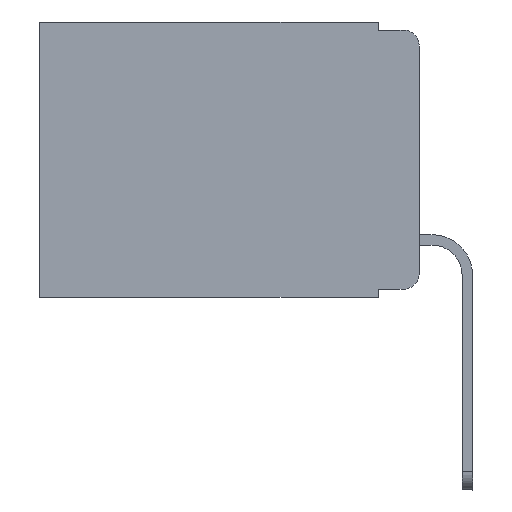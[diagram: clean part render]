
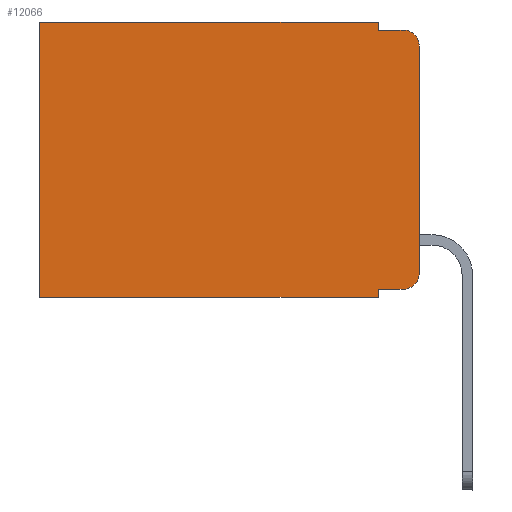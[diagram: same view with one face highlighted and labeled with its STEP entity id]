
A CAD part, left-side view. The second image highlights one B-rep face of the part: STEP entity #12066.
In plain terms, the highlighted planar face has unit normal (-1, 0, 0).
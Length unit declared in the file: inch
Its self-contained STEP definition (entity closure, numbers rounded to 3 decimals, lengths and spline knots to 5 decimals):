
#34 = CARTESIAN_POINT ( 'NONE',  ( 0.298, 0., 0. ) ) ;
#956 = EDGE_CURVE ( 'NONE', #10398, #2176, #9270, .T. ) ;
#1022 = VECTOR ( 'NONE', #3880, 39.37008 ) ;
#1063 = DIRECTION ( 'NONE',  ( 0., 0., -1. ) ) ;
#1098 = DIRECTION ( 'NONE',  ( 0., 0., -1. ) ) ;
#1176 = CARTESIAN_POINT ( 'NONE',  ( 0.298, 0.051, -0.333 ) ) ;
#1230 = ORIENTED_EDGE ( 'NONE', *, *, #5675, .T. ) ;
#1275 = VECTOR ( 'NONE', #1098, 39.37008 ) ;
#1310 = DIRECTION ( 'NONE',  ( 0., -1., 0. ) ) ;
#1517 = CARTESIAN_POINT ( 'NONE',  ( 0.298, 0.051, -0.333 ) ) ;
#1580 = CIRCLE ( 'NONE', #9011, 0.02 ) ;
#1820 = VERTEX_POINT ( 'NONE', #7042 ) ;
#1824 = ORIENTED_EDGE ( 'NONE', *, *, #9026, .F. ) ;
#1940 = DIRECTION ( 'NONE',  ( 0., 0., -1. ) ) ;
#2000 = EDGE_CURVE ( 'NONE', #2176, #11963, #5683, .T. ) ;
#2042 = CARTESIAN_POINT ( 'NONE',  ( 0.298, 0.051, 0. ) ) ;
#2048 = ORIENTED_EDGE ( 'NONE', *, *, #11549, .F. ) ;
#2062 = LINE ( 'NONE', #9158, #3409 ) ;
#2176 = VERTEX_POINT ( 'NONE', #4159 ) ;
#2185 = ORIENTED_EDGE ( 'NONE', *, *, #2980, .F. ) ;
#2361 = CARTESIAN_POINT ( 'NONE',  ( 0.298, 0.02, -0.03 ) ) ;
#2426 = CARTESIAN_POINT ( 'NONE',  ( 0.298, 0.02, -0.01 ) ) ;
#2501 = ORIENTED_EDGE ( 'NONE', *, *, #11627, .F. ) ;
#2846 = CARTESIAN_POINT ( 'NONE',  ( 0.298, 0.02, -0.313 ) ) ;
#2980 = EDGE_CURVE ( 'NONE', #12487, #12845, #4868, .T. ) ;
#3088 = LINE ( 'NONE', #1176, #11861 ) ;
#3409 = VECTOR ( 'NONE', #1063, 39.37008 ) ;
#3467 = CARTESIAN_POINT ( 'NONE',  ( 0.298, 0.051, -0.343 ) ) ;
#3501 = ORIENTED_EDGE ( 'NONE', *, *, #7907, .F. ) ;
#3747 = CARTESIAN_POINT ( 'NONE',  ( 0.298, 0., -0.343 ) ) ;
#3761 = DIRECTION ( 'NONE',  ( 0., 0., -1. ) ) ;
#3880 = DIRECTION ( 'NONE',  ( 0., -1., 0. ) ) ;
#3896 = EDGE_LOOP ( 'NONE', ( #3501, #8247, #2185, #1824, #11133, #9934, #2501, #2048, #1230, #10376 ) ) ;
#4099 = DIRECTION ( 'NONE',  ( -1., 0., 0. ) ) ;
#4159 = CARTESIAN_POINT ( 'NONE',  ( 0.298, 0.473, 0. ) ) ;
#4868 = LINE ( 'NONE', #12096, #1022 ) ;
#5112 = AXIS2_PLACEMENT_3D ( 'NONE', #5200, #9242, #12214 ) ;
#5200 = CARTESIAN_POINT ( 'NONE',  ( 0.298, 0., 0. ) ) ;
#5675 = EDGE_CURVE ( 'NONE', #12507, #10286, #3088, .T. ) ;
#5683 = LINE ( 'NONE', #9732, #12070 ) ;
#5734 = EDGE_CURVE ( 'NONE', #1820, #12845, #7430, .T. ) ;
#5740 = VECTOR ( 'NONE', #12167, 39.37008 ) ;
#5821 = VERTEX_POINT ( 'NONE', #3467 ) ;
#6168 = AXIS2_PLACEMENT_3D ( 'NONE', #2361, #7400, #6420 ) ;
#6203 = FACE_OUTER_BOUND ( 'NONE', #3896, .T. ) ;
#6230 = CARTESIAN_POINT ( 'NONE',  ( 0.298, 0., 0. ) ) ;
#6420 = DIRECTION ( 'NONE',  ( 0., 0., -1. ) ) ;
#6664 = EDGE_CURVE ( 'NONE', #10286, #10703, #1580, .T. ) ;
#7042 = CARTESIAN_POINT ( 'NONE',  ( 0.298, 0., -0.03 ) ) ;
#7080 = LINE ( 'NONE', #2042, #5740 ) ;
#7400 = DIRECTION ( 'NONE',  ( -1., 0., 0. ) ) ;
#7430 = CIRCLE ( 'NONE', #6168, 0.02 ) ;
#7816 = DIRECTION ( 'NONE',  ( 0., 1., 0. ) ) ;
#7907 = EDGE_CURVE ( 'NONE', #1820, #10703, #9119, .T. ) ;
#7977 = CARTESIAN_POINT ( 'NONE',  ( 0.298, 0., -0.313 ) ) ;
#8247 = ORIENTED_EDGE ( 'NONE', *, *, #5734, .T. ) ;
#8298 = VECTOR ( 'NONE', #7816, 39.37008 ) ;
#9011 = AXIS2_PLACEMENT_3D ( 'NONE', #2846, #4099, #1940 ) ;
#9026 = EDGE_CURVE ( 'NONE', #10398, #12487, #2062, .T. ) ;
#9119 = LINE ( 'NONE', #34, #1275 ) ;
#9158 = CARTESIAN_POINT ( 'NONE',  ( 0.298, 0.051, 0. ) ) ;
#9242 = DIRECTION ( 'NONE',  ( 1., 0., 0. ) ) ;
#9270 = LINE ( 'NONE', #6230, #12444 ) ;
#9439 = PLANE ( 'NONE',  #5112 ) ;
#9732 = CARTESIAN_POINT ( 'NONE',  ( 0.298, 0.473, 0. ) ) ;
#9934 = ORIENTED_EDGE ( 'NONE', *, *, #2000, .T. ) ;
#10063 = CARTESIAN_POINT ( 'NONE',  ( 0.298, 0.473, -0.343 ) ) ;
#10267 = DIRECTION ( 'NONE',  ( 0., 1., 0. ) ) ;
#10286 = VERTEX_POINT ( 'NONE', #11587 ) ;
#10376 = ORIENTED_EDGE ( 'NONE', *, *, #6664, .T. ) ;
#10398 = VERTEX_POINT ( 'NONE', #12539 ) ;
#10403 = CARTESIAN_POINT ( 'NONE',  ( 0.298, 0.051, -0.01 ) ) ;
#10703 = VERTEX_POINT ( 'NONE', #7977 ) ;
#11133 = ORIENTED_EDGE ( 'NONE', *, *, #956, .T. ) ;
#11549 = EDGE_CURVE ( 'NONE', #12507, #5821, #7080, .T. ) ;
#11587 = CARTESIAN_POINT ( 'NONE',  ( 0.298, 0.02, -0.333 ) ) ;
#11627 = EDGE_CURVE ( 'NONE', #5821, #11963, #12819, .T. ) ;
#11861 = VECTOR ( 'NONE', #1310, 39.37008 ) ;
#11963 = VERTEX_POINT ( 'NONE', #10063 ) ;
#12066 = ADVANCED_FACE ( 'NONE', ( #6203 ), #9439, .F. ) ;
#12070 = VECTOR ( 'NONE', #3761, 39.37008 ) ;
#12096 = CARTESIAN_POINT ( 'NONE',  ( 0.298, 0.051, -0.01 ) ) ;
#12167 = DIRECTION ( 'NONE',  ( 0., 0., -1. ) ) ;
#12214 = DIRECTION ( 'NONE',  ( 0., 0., -1. ) ) ;
#12444 = VECTOR ( 'NONE', #10267, 39.37008 ) ;
#12487 = VERTEX_POINT ( 'NONE', #10403 ) ;
#12507 = VERTEX_POINT ( 'NONE', #1517 ) ;
#12539 = CARTESIAN_POINT ( 'NONE',  ( 0.298, 0.051, 0. ) ) ;
#12819 = LINE ( 'NONE', #3747, #8298 ) ;
#12845 = VERTEX_POINT ( 'NONE', #2426 ) ;
